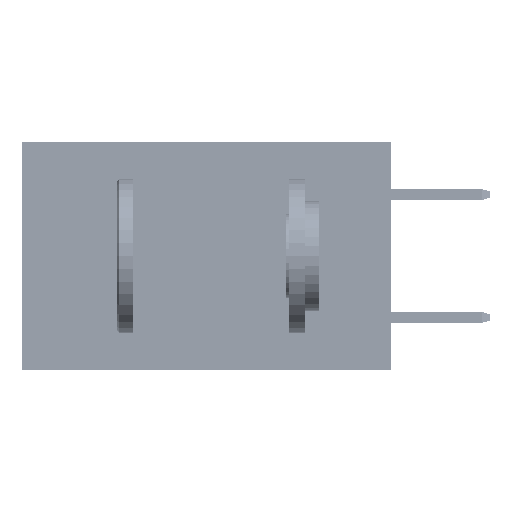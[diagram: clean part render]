
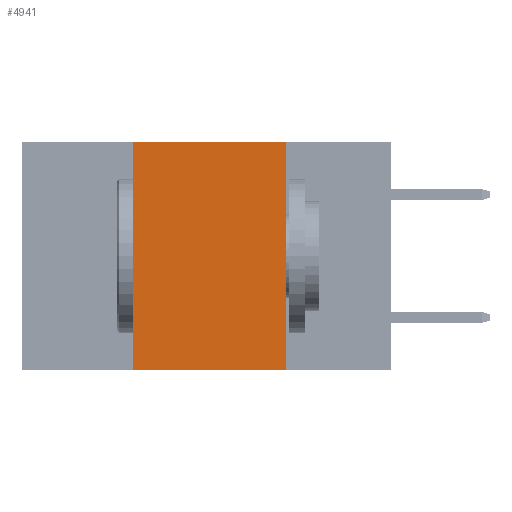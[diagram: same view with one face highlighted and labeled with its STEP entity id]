
A CAD part, left-side view. The second image highlights one B-rep face of the part: STEP entity #4941.
In plain terms, the highlighted planar face has unit normal (-1, 0, 0).
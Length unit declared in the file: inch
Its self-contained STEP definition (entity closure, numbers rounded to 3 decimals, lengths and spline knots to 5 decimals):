
#661 = DIRECTION ( 'NONE',  ( 0., 0., -1. ) ) ;
#3814 = CARTESIAN_POINT ( 'NONE',  ( 0., 0.6, -0.37 ) ) ;
#4941 = ADVANCED_FACE ( 'NONE', ( #24439 ), #29012, .F. ) ;
#5481 = CARTESIAN_POINT ( 'NONE',  ( 0., 0.6, 0. ) ) ;
#5648 = DIRECTION ( 'NONE',  ( 1., 0., 0. ) ) ;
#6938 = LINE ( 'NONE', #39435, #22932 ) ;
#7683 = LINE ( 'NONE', #3814, #14066 ) ;
#9423 = DIRECTION ( 'NONE',  ( 0., 0., -1. ) ) ;
#10423 = CARTESIAN_POINT ( 'NONE',  ( 0., 0.6, 0. ) ) ;
#12905 = VERTEX_POINT ( 'NONE', #28036 ) ;
#13289 = LINE ( 'NONE', #10423, #47648 ) ;
#14066 = VECTOR ( 'NONE', #19755, 39.37008 ) ;
#15871 = CARTESIAN_POINT ( 'NONE',  ( 0., 0.17, 0. ) ) ;
#15940 = EDGE_CURVE ( 'NONE', #20380, #12905, #6938, .T. ) ;
#17207 = CARTESIAN_POINT ( 'NONE',  ( 0., 0.42, 0. ) ) ;
#19755 = DIRECTION ( 'NONE',  ( 0., -1., 0. ) ) ;
#20380 = VERTEX_POINT ( 'NONE', #15871 ) ;
#22932 = VECTOR ( 'NONE', #661, 39.37008 ) ;
#23307 = ORIENTED_EDGE ( 'NONE', *, *, #15940, .F. ) ;
#24439 = FACE_OUTER_BOUND ( 'NONE', #40362, .T. ) ;
#24832 = EDGE_CURVE ( 'NONE', #40764, #20380, #13289, .T. ) ;
#28036 = CARTESIAN_POINT ( 'NONE',  ( 0., 0.17, -0.37 ) ) ;
#28626 = VERTEX_POINT ( 'NONE', #49921 ) ;
#29012 = PLANE ( 'NONE',  #48179 ) ;
#29753 = CARTESIAN_POINT ( 'NONE',  ( 0., 0.42, 0. ) ) ;
#33544 = VECTOR ( 'NONE', #37636, 39.37008 ) ;
#37348 = EDGE_CURVE ( 'NONE', #28626, #40764, #45197, .T. ) ;
#37636 = DIRECTION ( 'NONE',  ( 0., 0., 1. ) ) ;
#39435 = CARTESIAN_POINT ( 'NONE',  ( 0., 0.17, 0. ) ) ;
#40362 = EDGE_LOOP ( 'NONE', ( #23307, #44548, #42474, #48656 ) ) ;
#40764 = VERTEX_POINT ( 'NONE', #17207 ) ;
#42474 = ORIENTED_EDGE ( 'NONE', *, *, #37348, .F. ) ;
#44548 = ORIENTED_EDGE ( 'NONE', *, *, #24832, .F. ) ;
#45197 = LINE ( 'NONE', #29753, #33544 ) ;
#47648 = VECTOR ( 'NONE', #49342, 39.37008 ) ;
#48179 = AXIS2_PLACEMENT_3D ( 'NONE', #5481, #5648, #9423 ) ;
#48656 = ORIENTED_EDGE ( 'NONE', *, *, #49206, .T. ) ;
#49206 = EDGE_CURVE ( 'NONE', #28626, #12905, #7683, .T. ) ;
#49342 = DIRECTION ( 'NONE',  ( 0., -1., 0. ) ) ;
#49921 = CARTESIAN_POINT ( 'NONE',  ( 0., 0.42, -0.37 ) ) ;
